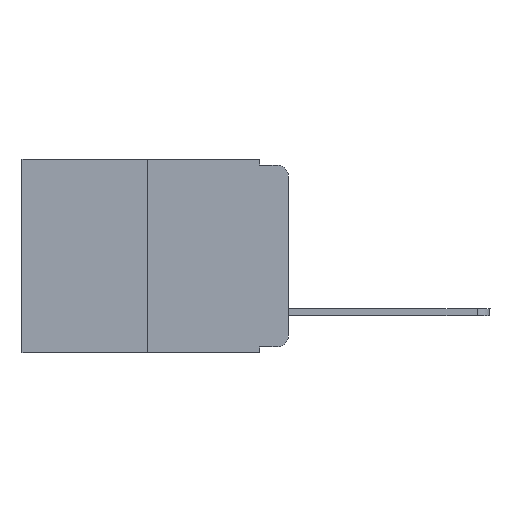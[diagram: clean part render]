
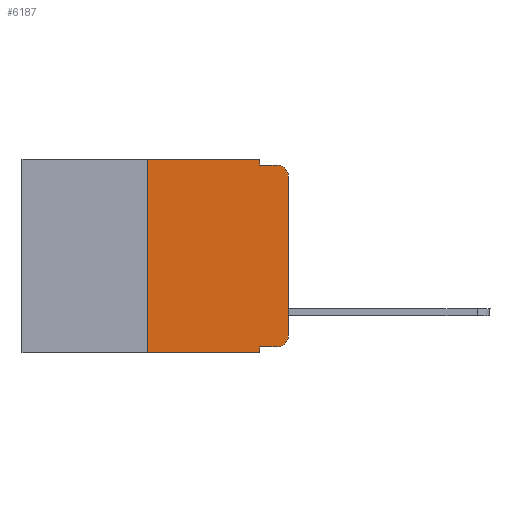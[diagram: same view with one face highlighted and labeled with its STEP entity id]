
A CAD part, left-side view. The second image highlights one B-rep face of the part: STEP entity #6187.
In plain terms, the highlighted planar face has unit normal (-1, 0, 0).
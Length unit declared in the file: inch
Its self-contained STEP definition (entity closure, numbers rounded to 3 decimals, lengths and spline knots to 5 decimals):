
#213 = CARTESIAN_POINT ( 'NONE',  ( 0., 0., -0.313 ) ) ;
#474 = DIRECTION ( 'NONE',  ( 0., -1., 0. ) ) ;
#481 = EDGE_CURVE ( 'NONE', #8569, #4959, #16549, .T. ) ;
#593 = EDGE_CURVE ( 'NONE', #10957, #2357, #17136, .T. ) ;
#899 = DIRECTION ( 'NONE',  ( 0., 0., -1. ) ) ;
#1278 = CARTESIAN_POINT ( 'NONE',  ( 0., 0.051, -0.333 ) ) ;
#1327 = EDGE_CURVE ( 'NONE', #4959, #2357, #6585, .T. ) ;
#2336 = VERTEX_POINT ( 'NONE', #4017 ) ;
#2357 = VERTEX_POINT ( 'NONE', #9644 ) ;
#2383 = VECTOR ( 'NONE', #15291, 39.37008 ) ;
#2424 = DIRECTION ( 'NONE',  ( 1., 0., 0. ) ) ;
#2453 = VECTOR ( 'NONE', #4800, 39.37008 ) ;
#2711 = DIRECTION ( 'NONE',  ( 0., 0., -1. ) ) ;
#2852 = ORIENTED_EDGE ( 'NONE', *, *, #18312, .T. ) ;
#3357 = EDGE_CURVE ( 'NONE', #4495, #2336, #10245, .T. ) ;
#3484 = CARTESIAN_POINT ( 'NONE',  ( 0., 0.051, -0.01 ) ) ;
#3582 = EDGE_CURVE ( 'NONE', #13687, #12028, #6403, .T. ) ;
#4017 = CARTESIAN_POINT ( 'NONE',  ( 0., 0.25, 0. ) ) ;
#4301 = EDGE_CURVE ( 'NONE', #2336, #8569, #7757, .T. ) ;
#4336 = CARTESIAN_POINT ( 'NONE',  ( 0., 0., -0.03 ) ) ;
#4495 = VERTEX_POINT ( 'NONE', #15960 ) ;
#4660 = LINE ( 'NONE', #15117, #14533 ) ;
#4800 = DIRECTION ( 'NONE',  ( 0., 0., 1. ) ) ;
#4942 = CARTESIAN_POINT ( 'NONE',  ( 0., 0.473, 0. ) ) ;
#4959 = VERTEX_POINT ( 'NONE', #10420 ) ;
#5436 = DIRECTION ( 'NONE',  ( 0., -1., 0. ) ) ;
#5473 = CARTESIAN_POINT ( 'NONE',  ( 0., 0.02, -0.313 ) ) ;
#5533 = LINE ( 'NONE', #1278, #8084 ) ;
#5575 = DIRECTION ( 'NONE',  ( 0., 0., -1. ) ) ;
#6118 = EDGE_LOOP ( 'NONE', ( #12584, #14364, #8195, #10346, #18920, #6835, #11845, #13482, #2852, #13792 ) ) ;
#6187 = ADVANCED_FACE ( 'NONE', ( #8712 ), #15864, .F. ) ;
#6403 = CIRCLE ( 'NONE', #11361, 0.02 ) ;
#6585 = LINE ( 'NONE', #3484, #2383 ) ;
#6835 = ORIENTED_EDGE ( 'NONE', *, *, #3357, .F. ) ;
#7434 = DIRECTION ( 'NONE',  ( 0., 0., 1. ) ) ;
#7473 = DIRECTION ( 'NONE',  ( 0., -1., 0. ) ) ;
#7628 = LINE ( 'NONE', #7734, #11445 ) ;
#7650 = VERTEX_POINT ( 'NONE', #13444 ) ;
#7734 = CARTESIAN_POINT ( 'NONE',  ( 0., 0.473, -0.343 ) ) ;
#7757 = LINE ( 'NONE', #4942, #18642 ) ;
#7865 = CARTESIAN_POINT ( 'NONE',  ( 0., 0.051, 0. ) ) ;
#8084 = VECTOR ( 'NONE', #5436, 39.37008 ) ;
#8152 = CARTESIAN_POINT ( 'NONE',  ( 0., 0.051, 0. ) ) ;
#8195 = ORIENTED_EDGE ( 'NONE', *, *, #1327, .F. ) ;
#8399 = VECTOR ( 'NONE', #18198, 39.37008 ) ;
#8569 = VERTEX_POINT ( 'NONE', #8152 ) ;
#8712 = FACE_OUTER_BOUND ( 'NONE', #6118, .T. ) ;
#9644 = CARTESIAN_POINT ( 'NONE',  ( 0., 0.02, -0.01 ) ) ;
#10245 = LINE ( 'NONE', #16134, #14477 ) ;
#10346 = ORIENTED_EDGE ( 'NONE', *, *, #481, .F. ) ;
#10420 = CARTESIAN_POINT ( 'NONE',  ( 0., 0.051, -0.01 ) ) ;
#10706 = CARTESIAN_POINT ( 'NONE',  ( 0., 0., 0. ) ) ;
#10957 = VERTEX_POINT ( 'NONE', #4336 ) ;
#11109 = EDGE_CURVE ( 'NONE', #12028, #10957, #14883, .T. ) ;
#11252 = DIRECTION ( 'NONE',  ( -1., 0., 0. ) ) ;
#11361 = AXIS2_PLACEMENT_3D ( 'NONE', #5473, #16990, #5575 ) ;
#11445 = VECTOR ( 'NONE', #474, 39.37008 ) ;
#11828 = CARTESIAN_POINT ( 'NONE',  ( 0., 0.02, -0.333 ) ) ;
#11845 = ORIENTED_EDGE ( 'NONE', *, *, #15491, .T. ) ;
#12007 = EDGE_CURVE ( 'NONE', #13200, #7650, #4660, .T. ) ;
#12028 = VERTEX_POINT ( 'NONE', #213 ) ;
#12584 = ORIENTED_EDGE ( 'NONE', *, *, #11109, .T. ) ;
#12783 = CARTESIAN_POINT ( 'NONE',  ( 0., 0.473, 0. ) ) ;
#13200 = VERTEX_POINT ( 'NONE', #14182 ) ;
#13444 = CARTESIAN_POINT ( 'NONE',  ( 0., 0.051, -0.343 ) ) ;
#13482 = ORIENTED_EDGE ( 'NONE', *, *, #12007, .F. ) ;
#13687 = VERTEX_POINT ( 'NONE', #11828 ) ;
#13792 = ORIENTED_EDGE ( 'NONE', *, *, #3582, .T. ) ;
#14182 = CARTESIAN_POINT ( 'NONE',  ( 0., 0.051, -0.333 ) ) ;
#14246 = CARTESIAN_POINT ( 'NONE',  ( 0., 0.02, -0.03 ) ) ;
#14364 = ORIENTED_EDGE ( 'NONE', *, *, #593, .T. ) ;
#14477 = VECTOR ( 'NONE', #7434, 39.37008 ) ;
#14533 = VECTOR ( 'NONE', #18002, 39.37008 ) ;
#14883 = LINE ( 'NONE', #10706, #2453 ) ;
#15117 = CARTESIAN_POINT ( 'NONE',  ( 0., 0.051, 0. ) ) ;
#15291 = DIRECTION ( 'NONE',  ( 0., -1., 0. ) ) ;
#15491 = EDGE_CURVE ( 'NONE', #4495, #7650, #7628, .T. ) ;
#15864 = PLANE ( 'NONE',  #17201 ) ;
#15960 = CARTESIAN_POINT ( 'NONE',  ( 0., 0.25, -0.343 ) ) ;
#16134 = CARTESIAN_POINT ( 'NONE',  ( 0., 0.25, 0. ) ) ;
#16549 = LINE ( 'NONE', #7865, #8399 ) ;
#16990 = DIRECTION ( 'NONE',  ( -1., 0., 0. ) ) ;
#17136 = CIRCLE ( 'NONE', #17755, 0.02 ) ;
#17201 = AXIS2_PLACEMENT_3D ( 'NONE', #12783, #2424, #2711 ) ;
#17755 = AXIS2_PLACEMENT_3D ( 'NONE', #14246, #11252, #899 ) ;
#18002 = DIRECTION ( 'NONE',  ( 0., 0., -1. ) ) ;
#18198 = DIRECTION ( 'NONE',  ( 0., 0., -1. ) ) ;
#18312 = EDGE_CURVE ( 'NONE', #13200, #13687, #5533, .T. ) ;
#18642 = VECTOR ( 'NONE', #7473, 39.37008 ) ;
#18920 = ORIENTED_EDGE ( 'NONE', *, *, #4301, .F. ) ;
